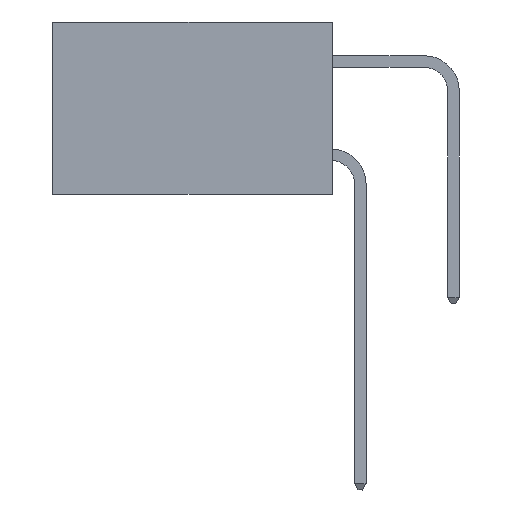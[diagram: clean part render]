
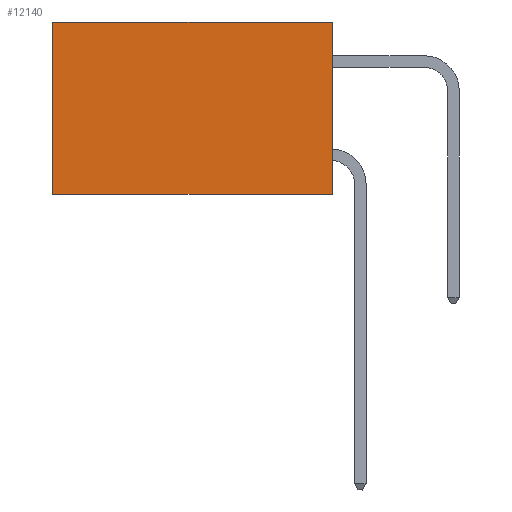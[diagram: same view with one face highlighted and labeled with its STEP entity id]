
A CAD part, left-side view. The second image highlights one B-rep face of the part: STEP entity #12140.
In plain terms, the highlighted planar face has unit normal (-1, 0, 0).
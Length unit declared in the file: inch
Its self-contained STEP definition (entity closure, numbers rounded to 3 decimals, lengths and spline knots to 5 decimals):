
#915 = ORIENTED_EDGE ( 'NONE', *, *, #5320, .T. ) ;
#1093 = CARTESIAN_POINT ( 'NONE',  ( 0.298, 0., 0. ) ) ;
#1702 = CARTESIAN_POINT ( 'NONE',  ( 0.298, 0., 0. ) ) ;
#1891 = VECTOR ( 'NONE', #9598, 39.37008 ) ;
#1971 = VECTOR ( 'NONE', #7053, 39.37008 ) ;
#2248 = DIRECTION ( 'NONE',  ( 0., 0., -1. ) ) ;
#2406 = CARTESIAN_POINT ( 'NONE',  ( 0.298, 0., 0. ) ) ;
#2602 = CARTESIAN_POINT ( 'NONE',  ( 0.298, 0.6, 0. ) ) ;
#3590 = EDGE_CURVE ( 'NONE', #9595, #6644, #7916, .T. ) ;
#3668 = CARTESIAN_POINT ( 'NONE',  ( 0.298, 0., 0. ) ) ;
#4241 = CARTESIAN_POINT ( 'NONE',  ( 0.298, 0., -0.37 ) ) ;
#4352 = FACE_OUTER_BOUND ( 'NONE', #7575, .T. ) ;
#5320 = EDGE_CURVE ( 'NONE', #6644, #9901, #13736, .T. ) ;
#6160 = CARTESIAN_POINT ( 'NONE',  ( 0.298, 0.6, -0.37 ) ) ;
#6237 = VERTEX_POINT ( 'NONE', #13016 ) ;
#6644 = VERTEX_POINT ( 'NONE', #6748 ) ;
#6748 = CARTESIAN_POINT ( 'NONE',  ( 0.298, 0.6, 0. ) ) ;
#6872 = DIRECTION ( 'NONE',  ( 1., 0., 0. ) ) ;
#7012 = DIRECTION ( 'NONE',  ( 0., 0., -1. ) ) ;
#7053 = DIRECTION ( 'NONE',  ( 0., 0., -1. ) ) ;
#7117 = EDGE_CURVE ( 'NONE', #6237, #9901, #12246, .T. ) ;
#7454 = EDGE_CURVE ( 'NONE', #9595, #6237, #7649, .T. ) ;
#7575 = EDGE_LOOP ( 'NONE', ( #915, #13069, #14689, #9916 ) ) ;
#7649 = LINE ( 'NONE', #3668, #1971 ) ;
#7916 = LINE ( 'NONE', #1702, #1891 ) ;
#8345 = VECTOR ( 'NONE', #11281, 39.37008 ) ;
#9595 = VERTEX_POINT ( 'NONE', #2406 ) ;
#9598 = DIRECTION ( 'NONE',  ( 0., 1., 0. ) ) ;
#9901 = VERTEX_POINT ( 'NONE', #6160 ) ;
#9916 = ORIENTED_EDGE ( 'NONE', *, *, #3590, .T. ) ;
#10688 = VECTOR ( 'NONE', #7012, 39.37008 ) ;
#11281 = DIRECTION ( 'NONE',  ( 0., 1., 0. ) ) ;
#11369 = PLANE ( 'NONE',  #13383 ) ;
#12140 = ADVANCED_FACE ( 'NONE', ( #4352 ), #11369, .F. ) ;
#12246 = LINE ( 'NONE', #4241, #8345 ) ;
#13016 = CARTESIAN_POINT ( 'NONE',  ( 0.298, 0., -0.37 ) ) ;
#13069 = ORIENTED_EDGE ( 'NONE', *, *, #7117, .F. ) ;
#13383 = AXIS2_PLACEMENT_3D ( 'NONE', #1093, #6872, #2248 ) ;
#13736 = LINE ( 'NONE', #2602, #10688 ) ;
#14689 = ORIENTED_EDGE ( 'NONE', *, *, #7454, .F. ) ;
